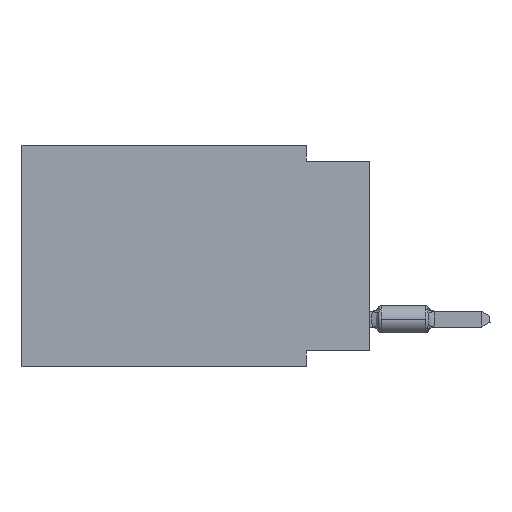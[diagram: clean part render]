
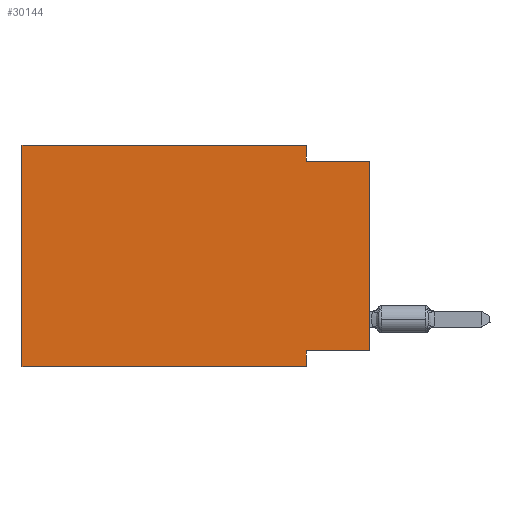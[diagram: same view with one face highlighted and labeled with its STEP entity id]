
A CAD part, left-side view. The second image highlights one B-rep face of the part: STEP entity #30144.
In plain terms, the highlighted planar face has unit normal (-1, 0, 0).
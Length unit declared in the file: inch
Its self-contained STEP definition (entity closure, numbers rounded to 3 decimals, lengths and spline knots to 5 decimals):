
#1402 = LINE ( 'NONE', #18650, #57718 ) ;
#1638 = VECTOR ( 'NONE', #23158, 39.37008 ) ;
#1707 = EDGE_CURVE ( 'NONE', #33482, #45849, #58500, .T. ) ;
#1861 = ORIENTED_EDGE ( 'NONE', *, *, #7102, .T. ) ;
#4156 = CARTESIAN_POINT ( 'NONE',  ( 0., 0.55, -0.35 ) ) ;
#4261 = DIRECTION ( 'NONE',  ( 0., 1., 0. ) ) ;
#5568 = CARTESIAN_POINT ( 'NONE',  ( 0., 0.1, -0.325 ) ) ;
#6439 = DIRECTION ( 'NONE',  ( 0., 0., -1. ) ) ;
#6741 = DIRECTION ( 'NONE',  ( 0., 0., -1. ) ) ;
#7102 = EDGE_CURVE ( 'NONE', #52525, #33676, #27054, .T. ) ;
#7316 = CARTESIAN_POINT ( 'NONE',  ( 0., 0.1, -0.35 ) ) ;
#8602 = DIRECTION ( 'NONE',  ( 0., -1., 0. ) ) ;
#8829 = CARTESIAN_POINT ( 'NONE',  ( 0., 0.55, 0. ) ) ;
#8901 = ORIENTED_EDGE ( 'NONE', *, *, #23232, .F. ) ;
#9038 = ORIENTED_EDGE ( 'NONE', *, *, #57126, .F. ) ;
#9446 = DIRECTION ( 'NONE',  ( 0., -1., 0. ) ) ;
#12288 = CARTESIAN_POINT ( 'NONE',  ( 0., 0., -0.325 ) ) ;
#12412 = EDGE_CURVE ( 'NONE', #52525, #27767, #22219, .T. ) ;
#13031 = CARTESIAN_POINT ( 'NONE',  ( 0., 0., -0.025 ) ) ;
#15641 = FACE_OUTER_BOUND ( 'NONE', #41650, .T. ) ;
#15852 = VERTEX_POINT ( 'NONE', #25901 ) ;
#15989 = CARTESIAN_POINT ( 'NONE',  ( 0., 0.1, -0.025 ) ) ;
#17806 = CARTESIAN_POINT ( 'NONE',  ( 0., 0., 0. ) ) ;
#18494 = VECTOR ( 'NONE', #57607, 39.37008 ) ;
#18565 = EDGE_CURVE ( 'NONE', #27767, #15852, #39508, .T. ) ;
#18650 = CARTESIAN_POINT ( 'NONE',  ( 0., 0., -0.025 ) ) ;
#20618 = CARTESIAN_POINT ( 'NONE',  ( 0., 0.55, 0. ) ) ;
#22219 = LINE ( 'NONE', #8829, #25943 ) ;
#22400 = ORIENTED_EDGE ( 'NONE', *, *, #25435, .F. ) ;
#23158 = DIRECTION ( 'NONE',  ( 0., 0., 1. ) ) ;
#23217 = CARTESIAN_POINT ( 'NONE',  ( 0., 0.55, -0.35 ) ) ;
#23232 = EDGE_CURVE ( 'NONE', #33482, #44790, #36356, .T. ) ;
#23869 = VERTEX_POINT ( 'NONE', #15989 ) ;
#25167 = LINE ( 'NONE', #51875, #36715 ) ;
#25435 = EDGE_CURVE ( 'NONE', #15852, #23869, #25167, .T. ) ;
#25901 = CARTESIAN_POINT ( 'NONE',  ( 0., 0.1, 0. ) ) ;
#25943 = VECTOR ( 'NONE', #40041, 39.37008 ) ;
#27054 = LINE ( 'NONE', #4156, #51092 ) ;
#27767 = VERTEX_POINT ( 'NONE', #20618 ) ;
#28781 = EDGE_CURVE ( 'NONE', #23869, #45849, #1402, .T. ) ;
#29343 = CARTESIAN_POINT ( 'NONE',  ( 0., 0.55, 0. ) ) ;
#30144 = ADVANCED_FACE ( 'NONE', ( #15641 ), #33790, .F. ) ;
#32018 = ORIENTED_EDGE ( 'NONE', *, *, #18565, .F. ) ;
#33482 = VERTEX_POINT ( 'NONE', #12288 ) ;
#33676 = VERTEX_POINT ( 'NONE', #37512 ) ;
#33790 = PLANE ( 'NONE',  #52098 ) ;
#34663 = LINE ( 'NONE', #7316, #35280 ) ;
#35280 = VECTOR ( 'NONE', #52756, 39.37008 ) ;
#36356 = LINE ( 'NONE', #53567, #50767 ) ;
#36715 = VECTOR ( 'NONE', #6439, 39.37008 ) ;
#37512 = CARTESIAN_POINT ( 'NONE',  ( 0., 0.1, -0.35 ) ) ;
#39508 = LINE ( 'NONE', #47522, #18494 ) ;
#40041 = DIRECTION ( 'NONE',  ( 0., 0., 1. ) ) ;
#41650 = EDGE_LOOP ( 'NONE', ( #48718, #52120, #22400, #32018, #47482, #1861, #9038, #8901 ) ) ;
#44790 = VERTEX_POINT ( 'NONE', #5568 ) ;
#45849 = VERTEX_POINT ( 'NONE', #13031 ) ;
#47434 = DIRECTION ( 'NONE',  ( 1., 0., 0. ) ) ;
#47482 = ORIENTED_EDGE ( 'NONE', *, *, #12412, .F. ) ;
#47522 = CARTESIAN_POINT ( 'NONE',  ( 0., 0.55, 0. ) ) ;
#48718 = ORIENTED_EDGE ( 'NONE', *, *, #1707, .T. ) ;
#50767 = VECTOR ( 'NONE', #4261, 39.37008 ) ;
#51092 = VECTOR ( 'NONE', #8602, 39.37008 ) ;
#51875 = CARTESIAN_POINT ( 'NONE',  ( 0., 0.1, 0. ) ) ;
#52098 = AXIS2_PLACEMENT_3D ( 'NONE', #29343, #47434, #6741 ) ;
#52120 = ORIENTED_EDGE ( 'NONE', *, *, #28781, .F. ) ;
#52525 = VERTEX_POINT ( 'NONE', #23217 ) ;
#52756 = DIRECTION ( 'NONE',  ( 0., 0., -1. ) ) ;
#53567 = CARTESIAN_POINT ( 'NONE',  ( 0., 0., -0.325 ) ) ;
#57126 = EDGE_CURVE ( 'NONE', #44790, #33676, #34663, .T. ) ;
#57607 = DIRECTION ( 'NONE',  ( 0., -1., 0. ) ) ;
#57718 = VECTOR ( 'NONE', #9446, 39.37008 ) ;
#58500 = LINE ( 'NONE', #17806, #1638 ) ;
